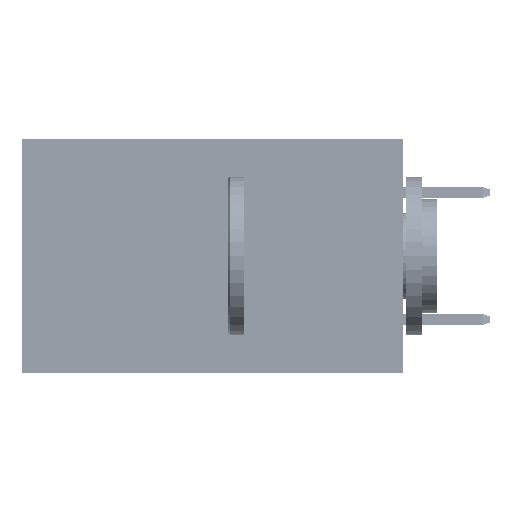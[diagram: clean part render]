
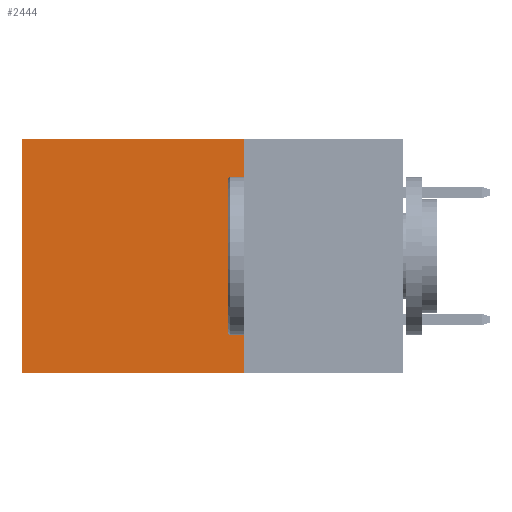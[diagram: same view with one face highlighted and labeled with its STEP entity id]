
A CAD part, left-side view. The second image highlights one B-rep face of the part: STEP entity #2444.
In plain terms, the highlighted planar face has unit normal (-1, 0, 0).
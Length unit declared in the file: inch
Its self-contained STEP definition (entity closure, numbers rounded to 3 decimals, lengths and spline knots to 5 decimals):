
#2444 = ADVANCED_FACE ( 'NONE', ( #4079 ), #19322, .F. ) ;
#4079 = FACE_OUTER_BOUND ( 'NONE', #18267, .T. ) ;
#4628 = VERTEX_POINT ( 'NONE', #7091 ) ;
#4757 = EDGE_CURVE ( 'NONE', #14342, #27845, #12082, .T. ) ;
#6803 = CARTESIAN_POINT ( 'NONE',  ( 0.2875, 0.25, 0. ) ) ;
#7091 = CARTESIAN_POINT ( 'NONE',  ( 0.2875, 0.25, -0.37 ) ) ;
#8090 = CARTESIAN_POINT ( 'NONE',  ( 0.2875, 0.25, 0. ) ) ;
#8155 = DIRECTION ( 'NONE',  ( 0., 1., 0. ) ) ;
#8871 = VECTOR ( 'NONE', #16086, 39.37008 ) ;
#11825 = ORIENTED_EDGE ( 'NONE', *, *, #45143, .T. ) ;
#12082 = LINE ( 'NONE', #8090, #8871 ) ;
#14342 = VERTEX_POINT ( 'NONE', #28993 ) ;
#14558 = CARTESIAN_POINT ( 'NONE',  ( 0.2875, 0.6, 0. ) ) ;
#15166 = LINE ( 'NONE', #34128, #26903 ) ;
#15579 = DIRECTION ( 'NONE',  ( 1., 0., 0. ) ) ;
#16086 = DIRECTION ( 'NONE',  ( 0., 1., 0. ) ) ;
#18267 = EDGE_LOOP ( 'NONE', ( #11825, #22048, #29422, #22978 ) ) ;
#18691 = CARTESIAN_POINT ( 'NONE',  ( 0.2875, 0.6, 0. ) ) ;
#19322 = PLANE ( 'NONE',  #20601 ) ;
#19751 = EDGE_CURVE ( 'NONE', #4628, #25542, #15166, .T. ) ;
#20601 = AXIS2_PLACEMENT_3D ( 'NONE', #34295, #15579, #38015 ) ;
#22048 = ORIENTED_EDGE ( 'NONE', *, *, #19751, .F. ) ;
#22978 = ORIENTED_EDGE ( 'NONE', *, *, #4757, .T. ) ;
#25542 = VERTEX_POINT ( 'NONE', #33878 ) ;
#26527 = VECTOR ( 'NONE', #33042, 39.37008 ) ;
#26903 = VECTOR ( 'NONE', #8155, 39.37008 ) ;
#27840 = EDGE_CURVE ( 'NONE', #14342, #4628, #37502, .T. ) ;
#27845 = VERTEX_POINT ( 'NONE', #14558 ) ;
#28993 = CARTESIAN_POINT ( 'NONE',  ( 0.2875, 0.25, 0. ) ) ;
#29246 = VECTOR ( 'NONE', #29703, 39.37008 ) ;
#29422 = ORIENTED_EDGE ( 'NONE', *, *, #27840, .F. ) ;
#29703 = DIRECTION ( 'NONE',  ( 0., 0., -1. ) ) ;
#33042 = DIRECTION ( 'NONE',  ( 0., 0., -1. ) ) ;
#33669 = LINE ( 'NONE', #18691, #29246 ) ;
#33878 = CARTESIAN_POINT ( 'NONE',  ( 0.2875, 0.6, -0.37 ) ) ;
#34128 = CARTESIAN_POINT ( 'NONE',  ( 0.2875, 0.25, -0.37 ) ) ;
#34295 = CARTESIAN_POINT ( 'NONE',  ( 0.2875, 0.25, 0. ) ) ;
#37502 = LINE ( 'NONE', #6803, #26527 ) ;
#38015 = DIRECTION ( 'NONE',  ( 0., 0., -1. ) ) ;
#45143 = EDGE_CURVE ( 'NONE', #27845, #25542, #33669, .T. ) ;
